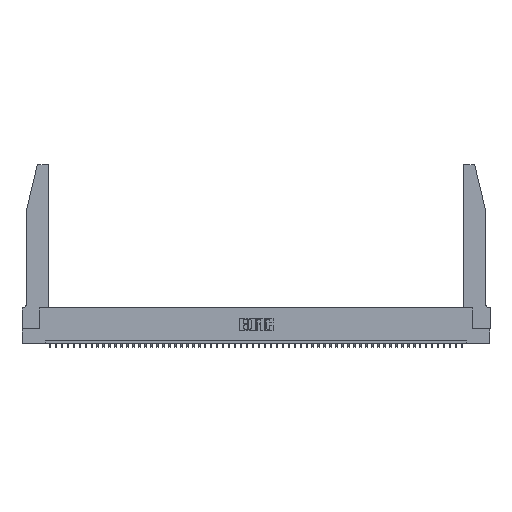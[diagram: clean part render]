
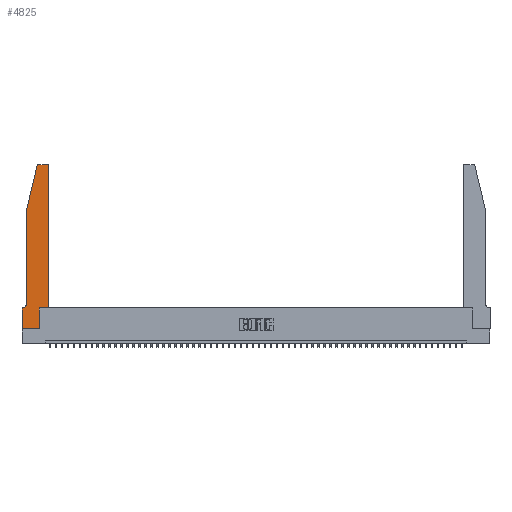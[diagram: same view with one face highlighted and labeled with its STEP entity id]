
A CAD part, top view. The second image highlights one B-rep face of the part: STEP entity #4825.
In plain terms, the highlighted planar face has unit normal (0, 0, 1).
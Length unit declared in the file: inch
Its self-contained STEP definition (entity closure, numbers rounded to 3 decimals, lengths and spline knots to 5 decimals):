
#535 = VERTEX_POINT ( 'NONE', #38169 ) ;
#1858 = VERTEX_POINT ( 'NONE', #16826 ) ;
#2250 = DIRECTION ( 'NONE',  ( 0., 1., 0. ) ) ;
#2587 = EDGE_CURVE ( 'NONE', #51514, #48043, #17141, .T. ) ;
#3401 = VECTOR ( 'NONE', #43572, 39.37008 ) ;
#4791 = DIRECTION ( 'NONE',  ( 0., 0., 1. ) ) ;
#4825 = ADVANCED_FACE ( 'NONE', ( #50009 ), #32921, .T. ) ;
#4900 = EDGE_CURVE ( 'NONE', #29018, #51514, #16893, .T. ) ;
#5068 = LINE ( 'NONE', #41107, #34386 ) ;
#7128 = VECTOR ( 'NONE', #18752, 39.37008 ) ;
#8981 = DIRECTION ( 'NONE',  ( 1., 0., 0. ) ) ;
#10006 = EDGE_LOOP ( 'NONE', ( #49354, #22842, #29250, #11598, #20516, #48188, #13040, #20002, #26739, #39815, #16281, #38031 ) ) ;
#10173 = CARTESIAN_POINT ( 'NONE',  ( 0.25487, 2.72718, 0.37 ) ) ;
#10525 = EDGE_CURVE ( 'NONE', #43026, #535, #43698, .T. ) ;
#11598 = ORIENTED_EDGE ( 'NONE', *, *, #4900, .T. ) ;
#13040 = ORIENTED_EDGE ( 'NONE', *, *, #45035, .T. ) ;
#13186 = VECTOR ( 'NONE', #2250, 39.37008 ) ;
#14490 = LINE ( 'NONE', #18610, #13186 ) ;
#15545 = DIRECTION ( 'NONE',  ( 0., 0., -1. ) ) ;
#15775 = CARTESIAN_POINT ( 'NONE',  ( 0.0755, 2., 0.37 ) ) ;
#16136 = CARTESIAN_POINT ( 'NONE',  ( 0., 0.35, 0.37 ) ) ;
#16281 = ORIENTED_EDGE ( 'NONE', *, *, #25113, .T. ) ;
#16826 = CARTESIAN_POINT ( 'NONE',  ( 0., 0., 0.37 ) ) ;
#16890 = EDGE_CURVE ( 'NONE', #34234, #37972, #14490, .T. ) ;
#16893 = LINE ( 'NONE', #15775, #26578 ) ;
#16942 = CARTESIAN_POINT ( 'NONE',  ( 0.4505, 2.72, 0.37 ) ) ;
#17141 = CIRCLE ( 'NONE', #30228, 0.07 ) ;
#17337 = VERTEX_POINT ( 'NONE', #44315 ) ;
#17929 = DIRECTION ( 'NONE',  ( 0., 1., 0. ) ) ;
#18610 = CARTESIAN_POINT ( 'NONE',  ( 0.2865, 0.35, 0.37 ) ) ;
#18752 = DIRECTION ( 'NONE',  ( 1., 0., 0. ) ) ;
#19638 = CARTESIAN_POINT ( 'NONE',  ( 0., 0., 0.37 ) ) ;
#20002 = ORIENTED_EDGE ( 'NONE', *, *, #31854, .T. ) ;
#20285 = DIRECTION ( 'NONE',  ( 1., 0., 0. ) ) ;
#20316 = EDGE_CURVE ( 'NONE', #535, #36554, #51198, .T. ) ;
#20516 = ORIENTED_EDGE ( 'NONE', *, *, #2587, .T. ) ;
#22842 = ORIENTED_EDGE ( 'NONE', *, *, #20316, .T. ) ;
#22994 = EDGE_CURVE ( 'NONE', #47917, #43026, #33012, .T. ) ;
#24773 = EDGE_CURVE ( 'NONE', #48043, #17337, #53010, .T. ) ;
#25113 = EDGE_CURVE ( 'NONE', #46425, #47917, #39263, .T. ) ;
#26578 = VECTOR ( 'NONE', #44830, 39.37008 ) ;
#26739 = ORIENTED_EDGE ( 'NONE', *, *, #16890, .T. ) ;
#26781 = VECTOR ( 'NONE', #28684, 39.37008 ) ;
#27867 = DIRECTION ( 'NONE',  ( 0., 0., 1. ) ) ;
#28248 = EDGE_CURVE ( 'NONE', #37972, #46425, #29247, .T. ) ;
#28419 = LINE ( 'NONE', #19638, #40792 ) ;
#28684 = DIRECTION ( 'NONE',  ( -1., 0., 0. ) ) ;
#28985 = CARTESIAN_POINT ( 'NONE',  ( 0.0755, 0.35, 0.37 ) ) ;
#29018 = VERTEX_POINT ( 'NONE', #53304 ) ;
#29247 = LINE ( 'NONE', #43866, #7128 ) ;
#29250 = ORIENTED_EDGE ( 'NONE', *, *, #43272, .T. ) ;
#29609 = VECTOR ( 'NONE', #34705, 39.37008 ) ;
#30228 = AXIS2_PLACEMENT_3D ( 'NONE', #32885, #15545, #33065 ) ;
#30528 = CARTESIAN_POINT ( 'NONE',  ( 0.0055, 0.35, 0.37 ) ) ;
#31674 = CARTESIAN_POINT ( 'NONE',  ( 0.284, 2.72, 0.37 ) ) ;
#31854 = EDGE_CURVE ( 'NONE', #1858, #34234, #37853, .T. ) ;
#32564 = CARTESIAN_POINT ( 'NONE',  ( 0.2865, 0., 0.37 ) ) ;
#32885 = CARTESIAN_POINT ( 'NONE',  ( 0.0055, 0.42, 0.37 ) ) ;
#32921 = PLANE ( 'NONE',  #34553 ) ;
#33012 = CIRCLE ( 'NONE', #53447, 0.03 ) ;
#33065 = DIRECTION ( 'NONE',  ( -1., 0., 0. ) ) ;
#34234 = VERTEX_POINT ( 'NONE', #32564 ) ;
#34386 = VECTOR ( 'NONE', #37305, 39.37008 ) ;
#34447 = CARTESIAN_POINT ( 'NONE',  ( 0.4205, 2.72, 0.37 ) ) ;
#34553 = AXIS2_PLACEMENT_3D ( 'NONE', #16136, #36719, #20285 ) ;
#34566 = CARTESIAN_POINT ( 'NONE',  ( 0.4505, 0.35, 0.37 ) ) ;
#34705 = DIRECTION ( 'NONE',  ( -1., 0., 0. ) ) ;
#36061 = DIRECTION ( 'NONE',  ( 1., 0., 0. ) ) ;
#36554 = VERTEX_POINT ( 'NONE', #10173 ) ;
#36719 = DIRECTION ( 'NONE',  ( 0., 0., 1. ) ) ;
#36805 = VECTOR ( 'NONE', #17929, 39.37008 ) ;
#37305 = DIRECTION ( 'NONE',  ( -0.239, -0.971, 0. ) ) ;
#37853 = LINE ( 'NONE', #45979, #3401 ) ;
#37972 = VERTEX_POINT ( 'NONE', #44616 ) ;
#38031 = ORIENTED_EDGE ( 'NONE', *, *, #22994, .T. ) ;
#38169 = CARTESIAN_POINT ( 'NONE',  ( 0.284, 2.75, 0.37 ) ) ;
#39263 = LINE ( 'NONE', #34566, #36805 ) ;
#39815 = ORIENTED_EDGE ( 'NONE', *, *, #28248, .T. ) ;
#39981 = CARTESIAN_POINT ( 'NONE',  ( 0.4205, 2.75, 0.37 ) ) ;
#40792 = VECTOR ( 'NONE', #43940, 39.37008 ) ;
#41107 = CARTESIAN_POINT ( 'NONE',  ( 0.0755, 2., 0.37 ) ) ;
#41286 = CARTESIAN_POINT ( 'NONE',  ( 0.4505, 0.35, 0.37 ) ) ;
#43026 = VERTEX_POINT ( 'NONE', #39981 ) ;
#43272 = EDGE_CURVE ( 'NONE', #36554, #29018, #5068, .T. ) ;
#43572 = DIRECTION ( 'NONE',  ( 1., 0., 0. ) ) ;
#43698 = LINE ( 'NONE', #53143, #26781 ) ;
#43866 = CARTESIAN_POINT ( 'NONE',  ( 0.4505, 0.35, 0.37 ) ) ;
#43940 = DIRECTION ( 'NONE',  ( 0., -1., 0. ) ) ;
#44315 = CARTESIAN_POINT ( 'NONE',  ( 0., 0.35, 0.37 ) ) ;
#44616 = CARTESIAN_POINT ( 'NONE',  ( 0.2865, 0.35, 0.37 ) ) ;
#44787 = AXIS2_PLACEMENT_3D ( 'NONE', #31674, #27867, #36061 ) ;
#44830 = DIRECTION ( 'NONE',  ( 0., -1., 0. ) ) ;
#45035 = EDGE_CURVE ( 'NONE', #17337, #1858, #28419, .T. ) ;
#45979 = CARTESIAN_POINT ( 'NONE',  ( 0., 0., 0.37 ) ) ;
#46425 = VERTEX_POINT ( 'NONE', #41286 ) ;
#46512 = CARTESIAN_POINT ( 'NONE',  ( 0.0755, 0.42, 0.37 ) ) ;
#47917 = VERTEX_POINT ( 'NONE', #16942 ) ;
#48043 = VERTEX_POINT ( 'NONE', #30528 ) ;
#48188 = ORIENTED_EDGE ( 'NONE', *, *, #24773, .T. ) ;
#49354 = ORIENTED_EDGE ( 'NONE', *, *, #10525, .T. ) ;
#50009 = FACE_OUTER_BOUND ( 'NONE', #10006, .T. ) ;
#51198 = CIRCLE ( 'NONE', #44787, 0.03 ) ;
#51514 = VERTEX_POINT ( 'NONE', #46512 ) ;
#53010 = LINE ( 'NONE', #28985, #29609 ) ;
#53143 = CARTESIAN_POINT ( 'NONE',  ( 0.2605, 2.75, 0.37 ) ) ;
#53304 = CARTESIAN_POINT ( 'NONE',  ( 0.0755, 2., 0.37 ) ) ;
#53447 = AXIS2_PLACEMENT_3D ( 'NONE', #34447, #4791, #8981 ) ;
